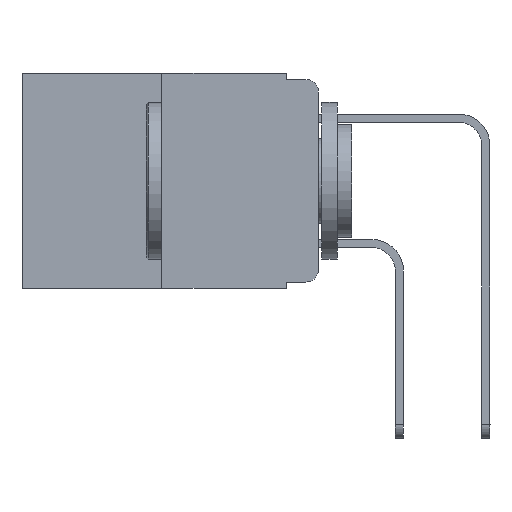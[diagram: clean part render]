
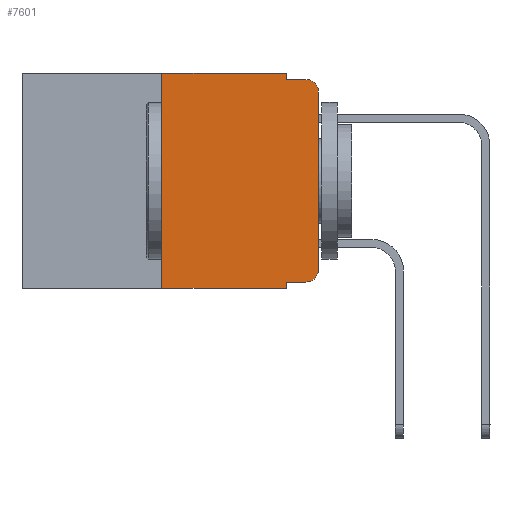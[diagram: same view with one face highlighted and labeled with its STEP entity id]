
A CAD part, left-side view. The second image highlights one B-rep face of the part: STEP entity #7601.
In plain terms, the highlighted planar face has unit normal (-1, 0, 0).
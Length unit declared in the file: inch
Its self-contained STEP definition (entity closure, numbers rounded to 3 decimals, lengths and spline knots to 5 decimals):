
#2 = ORIENTED_EDGE ( 'NONE', *, *, #16395, .T. ) ;
#929 = DIRECTION ( 'NONE',  ( 0., 0., -1. ) ) ;
#931 = VERTEX_POINT ( 'NONE', #13389 ) ;
#1097 = VERTEX_POINT ( 'NONE', #14105 ) ;
#1142 = EDGE_CURVE ( 'NONE', #6527, #5609, #9743, .T. ) ;
#1275 = DIRECTION ( 'NONE',  ( 0., -1., 0. ) ) ;
#1412 = CARTESIAN_POINT ( 'NONE',  ( 0., 0.051, 0. ) ) ;
#1434 = VERTEX_POINT ( 'NONE', #17975 ) ;
#1643 = DIRECTION ( 'NONE',  ( 0., -1., 0. ) ) ;
#1999 = DIRECTION ( 'NONE',  ( 0., 0., 1. ) ) ;
#2699 = DIRECTION ( 'NONE',  ( 1., 0., 0. ) ) ;
#3444 = DIRECTION ( 'NONE',  ( 0., 0., -1. ) ) ;
#3514 = CARTESIAN_POINT ( 'NONE',  ( 0., 0.25, 0. ) ) ;
#4593 = VERTEX_POINT ( 'NONE', #15921 ) ;
#4767 = DIRECTION ( 'NONE',  ( 0., -1., 0. ) ) ;
#5037 = CARTESIAN_POINT ( 'NONE',  ( 0., 0.473, -0.343 ) ) ;
#5456 = LINE ( 'NONE', #1412, #8031 ) ;
#5607 = VECTOR ( 'NONE', #1643, 39.37008 ) ;
#5609 = VERTEX_POINT ( 'NONE', #14563 ) ;
#5885 = CIRCLE ( 'NONE', #21067, 0.02 ) ;
#6175 = LINE ( 'NONE', #14723, #15895 ) ;
#6527 = VERTEX_POINT ( 'NONE', #23079 ) ;
#7601 = ADVANCED_FACE ( 'NONE', ( #26082 ), #8718, .F. ) ;
#7781 = CARTESIAN_POINT ( 'NONE',  ( 0., 0.051, 0. ) ) ;
#7807 = VERTEX_POINT ( 'NONE', #20463 ) ;
#8031 = VECTOR ( 'NONE', #24936, 39.37008 ) ;
#8050 = ORIENTED_EDGE ( 'NONE', *, *, #17463, .F. ) ;
#8718 = PLANE ( 'NONE',  #16133 ) ;
#9743 = LINE ( 'NONE', #20807, #5607 ) ;
#9944 = LINE ( 'NONE', #20726, #22065 ) ;
#10523 = CARTESIAN_POINT ( 'NONE',  ( 0., 0.25, -0.343 ) ) ;
#11226 = EDGE_CURVE ( 'NONE', #1434, #20733, #5885, .T. ) ;
#12213 = CARTESIAN_POINT ( 'NONE',  ( 0., 0.02, -0.03 ) ) ;
#12522 = VERTEX_POINT ( 'NONE', #16039 ) ;
#12533 = EDGE_CURVE ( 'NONE', #6527, #1097, #16333, .T. ) ;
#13389 = CARTESIAN_POINT ( 'NONE',  ( 0., 0.051, 0. ) ) ;
#13551 = ORIENTED_EDGE ( 'NONE', *, *, #12533, .F. ) ;
#13668 = CARTESIAN_POINT ( 'NONE',  ( 0., 0.02, -0.313 ) ) ;
#13858 = VECTOR ( 'NONE', #27177, 39.37008 ) ;
#13895 = ORIENTED_EDGE ( 'NONE', *, *, #19798, .T. ) ;
#14105 = CARTESIAN_POINT ( 'NONE',  ( 0., 0.051, -0.343 ) ) ;
#14563 = CARTESIAN_POINT ( 'NONE',  ( 0., 0.02, -0.333 ) ) ;
#14600 = DIRECTION ( 'NONE',  ( -1., 0., 0. ) ) ;
#14723 = CARTESIAN_POINT ( 'NONE',  ( 0., 0., 0. ) ) ;
#14884 = VECTOR ( 'NONE', #3444, 39.37008 ) ;
#15419 = LINE ( 'NONE', #5037, #22002 ) ;
#15895 = VECTOR ( 'NONE', #1999, 39.37008 ) ;
#15921 = CARTESIAN_POINT ( 'NONE',  ( 0., 0.25, 0. ) ) ;
#16039 = CARTESIAN_POINT ( 'NONE',  ( 0., 0.051, -0.01 ) ) ;
#16125 = ORIENTED_EDGE ( 'NONE', *, *, #1142, .T. ) ;
#16133 = AXIS2_PLACEMENT_3D ( 'NONE', #19380, #2699, #19645 ) ;
#16333 = LINE ( 'NONE', #7781, #14884 ) ;
#16395 = EDGE_CURVE ( 'NONE', #21128, #1097, #15419, .T. ) ;
#17313 = CARTESIAN_POINT ( 'NONE',  ( 0., 0.473, 0. ) ) ;
#17463 = EDGE_CURVE ( 'NONE', #4593, #931, #25723, .T. ) ;
#17975 = CARTESIAN_POINT ( 'NONE',  ( 0., 0., -0.03 ) ) ;
#17987 = EDGE_CURVE ( 'NONE', #12522, #20733, #9944, .T. ) ;
#19380 = CARTESIAN_POINT ( 'NONE',  ( 0., 0.473, 0. ) ) ;
#19496 = ORIENTED_EDGE ( 'NONE', *, *, #17987, .F. ) ;
#19522 = CARTESIAN_POINT ( 'NONE',  ( 0., 0.02, -0.01 ) ) ;
#19645 = DIRECTION ( 'NONE',  ( 0., 0., -1. ) ) ;
#19798 = EDGE_CURVE ( 'NONE', #7807, #1434, #6175, .T. ) ;
#20253 = VECTOR ( 'NONE', #23752, 39.37008 ) ;
#20463 = CARTESIAN_POINT ( 'NONE',  ( 0., 0., -0.313 ) ) ;
#20534 = ORIENTED_EDGE ( 'NONE', *, *, #21421, .F. ) ;
#20726 = CARTESIAN_POINT ( 'NONE',  ( 0., 0.051, -0.01 ) ) ;
#20733 = VERTEX_POINT ( 'NONE', #19522 ) ;
#20807 = CARTESIAN_POINT ( 'NONE',  ( 0., 0.051, -0.333 ) ) ;
#21065 = CIRCLE ( 'NONE', #24213, 0.02 ) ;
#21067 = AXIS2_PLACEMENT_3D ( 'NONE', #12213, #14600, #22718 ) ;
#21128 = VERTEX_POINT ( 'NONE', #10523 ) ;
#21301 = EDGE_CURVE ( 'NONE', #931, #12522, #5456, .T. ) ;
#21421 = EDGE_CURVE ( 'NONE', #21128, #4593, #24648, .T. ) ;
#22002 = VECTOR ( 'NONE', #4767, 39.37008 ) ;
#22065 = VECTOR ( 'NONE', #1275, 39.37008 ) ;
#22148 = ORIENTED_EDGE ( 'NONE', *, *, #11226, .T. ) ;
#22718 = DIRECTION ( 'NONE',  ( 0., 0., -1. ) ) ;
#22964 = EDGE_CURVE ( 'NONE', #5609, #7807, #21065, .T. ) ;
#23079 = CARTESIAN_POINT ( 'NONE',  ( 0., 0.051, -0.333 ) ) ;
#23533 = EDGE_LOOP ( 'NONE', ( #13895, #22148, #19496, #25878, #8050, #20534, #2, #13551, #16125, #23638 ) ) ;
#23638 = ORIENTED_EDGE ( 'NONE', *, *, #22964, .T. ) ;
#23752 = DIRECTION ( 'NONE',  ( 0., -1., 0. ) ) ;
#23797 = DIRECTION ( 'NONE',  ( -1., 0., 0. ) ) ;
#24213 = AXIS2_PLACEMENT_3D ( 'NONE', #13668, #23797, #929 ) ;
#24648 = LINE ( 'NONE', #3514, #13858 ) ;
#24936 = DIRECTION ( 'NONE',  ( 0., 0., -1. ) ) ;
#25723 = LINE ( 'NONE', #17313, #20253 ) ;
#25878 = ORIENTED_EDGE ( 'NONE', *, *, #21301, .F. ) ;
#26082 = FACE_OUTER_BOUND ( 'NONE', #23533, .T. ) ;
#27177 = DIRECTION ( 'NONE',  ( 0., 0., 1. ) ) ;
